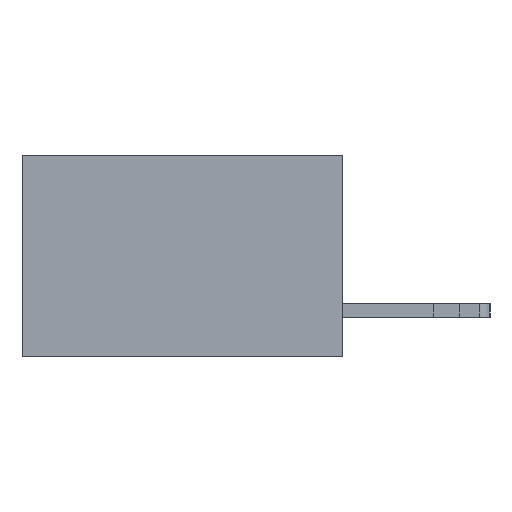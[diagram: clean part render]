
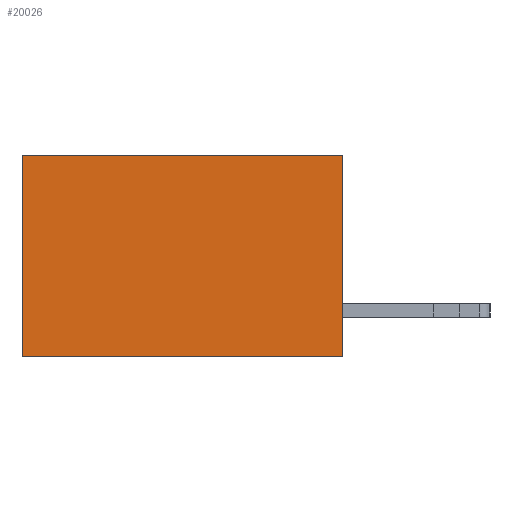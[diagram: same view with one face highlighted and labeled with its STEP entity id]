
A CAD part, left-side view. The second image highlights one B-rep face of the part: STEP entity #20026.
In plain terms, the highlighted planar face has unit normal (-1, 0, 0).
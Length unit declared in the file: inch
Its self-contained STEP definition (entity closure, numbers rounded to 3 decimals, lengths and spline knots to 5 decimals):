
#388 = CARTESIAN_POINT ( 'NONE',  ( 0.277, 0., 0. ) ) ;
#1261 = VERTEX_POINT ( 'NONE', #3316 ) ;
#1625 = EDGE_CURVE ( 'NONE', #9754, #20230, #4275, .T. ) ;
#2513 = DIRECTION ( 'NONE',  ( 0., 0., -1. ) ) ;
#2531 = VECTOR ( 'NONE', #16123, 39.37008 ) ;
#2538 = CARTESIAN_POINT ( 'NONE',  ( 0.277, 0., -0.37 ) ) ;
#2908 = ORIENTED_EDGE ( 'NONE', *, *, #1625, .F. ) ;
#3316 = CARTESIAN_POINT ( 'NONE',  ( 0.277, 0.59, 0. ) ) ;
#3349 = CARTESIAN_POINT ( 'NONE',  ( 0.277, 0., -0.37 ) ) ;
#3478 = CARTESIAN_POINT ( 'NONE',  ( 0.277, 0.59, -0.37 ) ) ;
#3489 = ORIENTED_EDGE ( 'NONE', *, *, #4577, .F. ) ;
#3503 = LINE ( 'NONE', #2538, #13645 ) ;
#4275 = LINE ( 'NONE', #22414, #22712 ) ;
#4470 = VERTEX_POINT ( 'NONE', #388 ) ;
#4577 = EDGE_CURVE ( 'NONE', #4470, #9754, #3503, .T. ) ;
#5169 = DIRECTION ( 'NONE',  ( 0., 1., 0. ) ) ;
#5185 = DIRECTION ( 'NONE',  ( 1., 0., 0. ) ) ;
#5745 = CARTESIAN_POINT ( 'NONE',  ( 0.277, 0., -0.37 ) ) ;
#8013 = AXIS2_PLACEMENT_3D ( 'NONE', #3349, #5185, #17830 ) ;
#8131 = DIRECTION ( 'NONE',  ( 0., 1., 0. ) ) ;
#8320 = ORIENTED_EDGE ( 'NONE', *, *, #22431, .T. ) ;
#9743 = EDGE_LOOP ( 'NONE', ( #21457, #2908, #3489, #8320 ) ) ;
#9754 = VERTEX_POINT ( 'NONE', #5745 ) ;
#10137 = VECTOR ( 'NONE', #8131, 39.37008 ) ;
#13645 = VECTOR ( 'NONE', #2513, 39.37008 ) ;
#13801 = LINE ( 'NONE', #18931, #10137 ) ;
#14070 = PLANE ( 'NONE',  #8013 ) ;
#16123 = DIRECTION ( 'NONE',  ( 0., 0., -1. ) ) ;
#17470 = EDGE_CURVE ( 'NONE', #1261, #20230, #20562, .T. ) ;
#17830 = DIRECTION ( 'NONE',  ( 0., 0., -1. ) ) ;
#18440 = CARTESIAN_POINT ( 'NONE',  ( 0.277, 0.59, -0.37 ) ) ;
#18931 = CARTESIAN_POINT ( 'NONE',  ( 0.277, 0., 0. ) ) ;
#20026 = ADVANCED_FACE ( 'NONE', ( #20947 ), #14070, .F. ) ;
#20230 = VERTEX_POINT ( 'NONE', #18440 ) ;
#20562 = LINE ( 'NONE', #3478, #2531 ) ;
#20947 = FACE_OUTER_BOUND ( 'NONE', #9743, .T. ) ;
#21457 = ORIENTED_EDGE ( 'NONE', *, *, #17470, .T. ) ;
#22414 = CARTESIAN_POINT ( 'NONE',  ( 0.277, 0., -0.37 ) ) ;
#22431 = EDGE_CURVE ( 'NONE', #4470, #1261, #13801, .T. ) ;
#22712 = VECTOR ( 'NONE', #5169, 39.37008 ) ;
